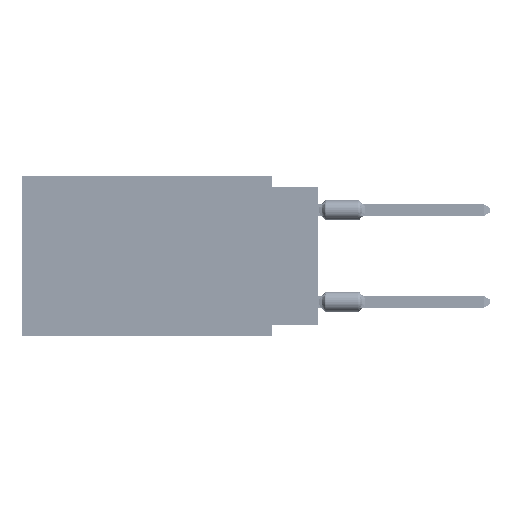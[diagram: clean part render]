
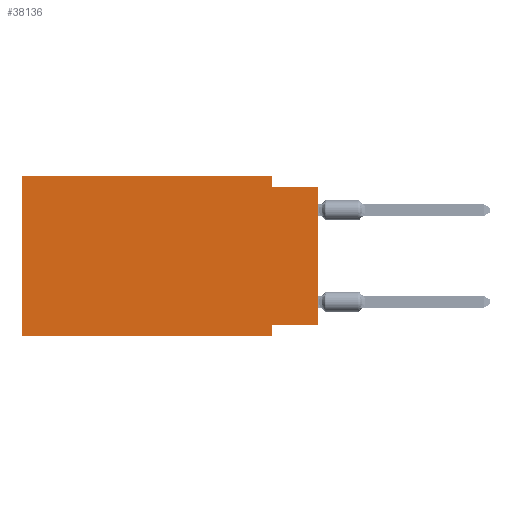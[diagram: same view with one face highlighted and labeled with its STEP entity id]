
A CAD part, left-side view. The second image highlights one B-rep face of the part: STEP entity #38136.
In plain terms, the highlighted planar face has unit normal (-1, 0, 0).
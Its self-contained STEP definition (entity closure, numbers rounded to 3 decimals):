
#3077 = DIRECTION ( 'NONE',  ( 0., 1., 0. ) ) ;
#4245 = VERTEX_POINT ( 'NONE', #4559 ) ;
#4559 = CARTESIAN_POINT ( 'NONE',  ( 0., 2.54, -8.89 ) ) ;
#4900 = DIRECTION ( 'NONE',  ( 0., -1., 0. ) ) ;
#5140 = LINE ( 'NONE', #68097, #16475 ) ;
#5343 = CARTESIAN_POINT ( 'NONE',  ( 0., 0., -0.635 ) ) ;
#7199 = VECTOR ( 'NONE', #20243, 1000. ) ;
#7399 = CARTESIAN_POINT ( 'NONE',  ( 0., 16.383, -8.89 ) ) ;
#7438 = ORIENTED_EDGE ( 'NONE', *, *, #38712, .F. ) ;
#8150 = LINE ( 'NONE', #22413, #55113 ) ;
#9336 = ORIENTED_EDGE ( 'NONE', *, *, #22100, .T. ) ;
#9853 = ORIENTED_EDGE ( 'NONE', *, *, #78700, .F. ) ;
#9932 = CARTESIAN_POINT ( 'NONE',  ( 0., 2.54, -8.255 ) ) ;
#10495 = FACE_OUTER_BOUND ( 'NONE', #81369, .T. ) ;
#11180 = VERTEX_POINT ( 'NONE', #17554 ) ;
#12307 = DIRECTION ( 'NONE',  ( 0., 0., -1. ) ) ;
#12989 = LINE ( 'NONE', #19442, #55062 ) ;
#14678 = ORIENTED_EDGE ( 'NONE', *, *, #59888, .F. ) ;
#15398 = VECTOR ( 'NONE', #35581, 1000. ) ;
#15647 = VERTEX_POINT ( 'NONE', #47063 ) ;
#16475 = VECTOR ( 'NONE', #26278, 1000. ) ;
#17375 = EDGE_CURVE ( 'NONE', #36598, #80553, #5140, .T. ) ;
#17513 = VERTEX_POINT ( 'NONE', #7399 ) ;
#17554 = CARTESIAN_POINT ( 'NONE',  ( 0., 16.383, 0. ) ) ;
#18721 = CARTESIAN_POINT ( 'NONE',  ( 0., 2.54, -0.635 ) ) ;
#19442 = CARTESIAN_POINT ( 'NONE',  ( 0., 16.383, -8.89 ) ) ;
#20243 = DIRECTION ( 'NONE',  ( 0., 0., -1. ) ) ;
#22100 = EDGE_CURVE ( 'NONE', #17513, #4245, #12989, .T. ) ;
#22413 = CARTESIAN_POINT ( 'NONE',  ( 0., 0., -8.255 ) ) ;
#25738 = ORIENTED_EDGE ( 'NONE', *, *, #17375, .T. ) ;
#26278 = DIRECTION ( 'NONE',  ( 0., 0., 1. ) ) ;
#27121 = CARTESIAN_POINT ( 'NONE',  ( 0., 2.54, 0. ) ) ;
#29745 = EDGE_CURVE ( 'NONE', #11180, #15647, #88057, .T. ) ;
#35581 = DIRECTION ( 'NONE',  ( 0., 0., 1. ) ) ;
#36487 = VECTOR ( 'NONE', #62286, 1000. ) ;
#36598 = VERTEX_POINT ( 'NONE', #38269 ) ;
#37162 = VERTEX_POINT ( 'NONE', #18721 ) ;
#38136 = ADVANCED_FACE ( 'NONE', ( #10495 ), #38538, .F. ) ;
#38269 = CARTESIAN_POINT ( 'NONE',  ( 0., 0., -8.255 ) ) ;
#38538 = PLANE ( 'NONE',  #45229 ) ;
#38712 = EDGE_CURVE ( 'NONE', #73250, #4245, #48502, .T. ) ;
#40347 = DIRECTION ( 'NONE',  ( 1., 0., 0. ) ) ;
#42467 = LINE ( 'NONE', #69153, #15398 ) ;
#45229 = AXIS2_PLACEMENT_3D ( 'NONE', #47686, #40347, #12307 ) ;
#47063 = CARTESIAN_POINT ( 'NONE',  ( 0., 2.54, 0. ) ) ;
#47686 = CARTESIAN_POINT ( 'NONE',  ( 0., 16.383, 0. ) ) ;
#48155 = VECTOR ( 'NONE', #59593, 1000. ) ;
#48502 = LINE ( 'NONE', #54943, #36487 ) ;
#51286 = LINE ( 'NONE', #27121, #7199 ) ;
#53982 = ORIENTED_EDGE ( 'NONE', *, *, #85647, .F. ) ;
#54943 = CARTESIAN_POINT ( 'NONE',  ( 0., 2.54, -8.89 ) ) ;
#55056 = ORIENTED_EDGE ( 'NONE', *, *, #29745, .F. ) ;
#55062 = VECTOR ( 'NONE', #75050, 1000. ) ;
#55113 = VECTOR ( 'NONE', #3077, 1000. ) ;
#59593 = DIRECTION ( 'NONE',  ( 0., -1., 0. ) ) ;
#59888 = EDGE_CURVE ( 'NONE', #15647, #37162, #51286, .T. ) ;
#60264 = CARTESIAN_POINT ( 'NONE',  ( 0., 0., -0.635 ) ) ;
#62286 = DIRECTION ( 'NONE',  ( 0., 0., -1. ) ) ;
#65434 = VECTOR ( 'NONE', #4900, 1000. ) ;
#68097 = CARTESIAN_POINT ( 'NONE',  ( 0., 0., 0. ) ) ;
#69153 = CARTESIAN_POINT ( 'NONE',  ( 0., 16.383, 0. ) ) ;
#72843 = ORIENTED_EDGE ( 'NONE', *, *, #82862, .F. ) ;
#73250 = VERTEX_POINT ( 'NONE', #9932 ) ;
#73825 = CARTESIAN_POINT ( 'NONE',  ( 0., 16.383, 0. ) ) ;
#75050 = DIRECTION ( 'NONE',  ( 0., -1., 0. ) ) ;
#75204 = LINE ( 'NONE', #5343, #65434 ) ;
#78700 = EDGE_CURVE ( 'NONE', #17513, #11180, #42467, .T. ) ;
#80553 = VERTEX_POINT ( 'NONE', #60264 ) ;
#81369 = EDGE_LOOP ( 'NONE', ( #25738, #53982, #14678, #55056, #9853, #9336, #7438, #72843 ) ) ;
#82862 = EDGE_CURVE ( 'NONE', #36598, #73250, #8150, .T. ) ;
#85647 = EDGE_CURVE ( 'NONE', #37162, #80553, #75204, .T. ) ;
#88057 = LINE ( 'NONE', #73825, #48155 ) ;
